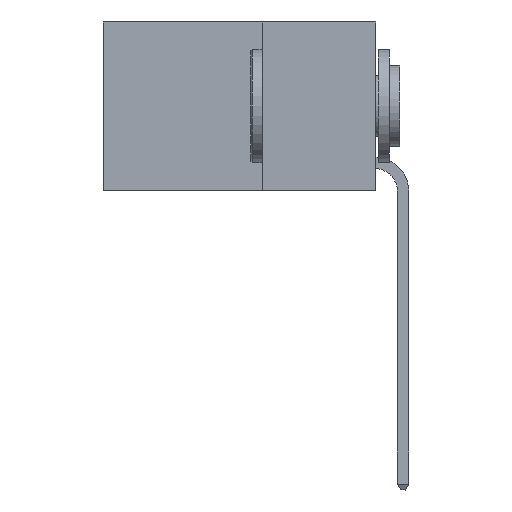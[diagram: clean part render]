
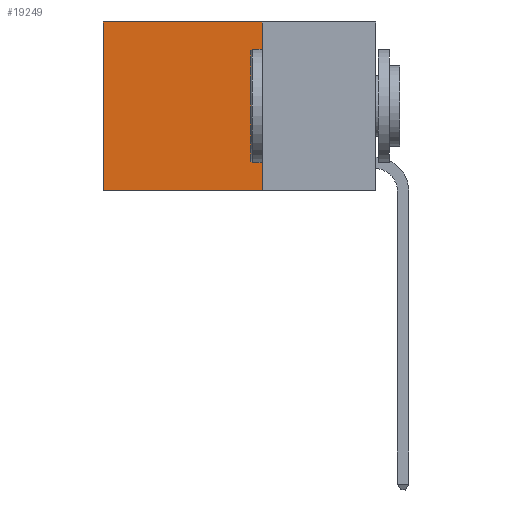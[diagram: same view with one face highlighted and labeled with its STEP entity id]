
A CAD part, left-side view. The second image highlights one B-rep face of the part: STEP entity #19249.
In plain terms, the highlighted planar face has unit normal (-1, 0, 0).
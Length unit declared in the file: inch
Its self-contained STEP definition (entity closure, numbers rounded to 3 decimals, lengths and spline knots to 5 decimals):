
#823 = VECTOR ( 'NONE', #17394, 39.37008 ) ;
#1607 = CARTESIAN_POINT ( 'NONE',  ( 0.2625, 0.25, -0.37 ) ) ;
#2812 = CARTESIAN_POINT ( 'NONE',  ( 0.2625, 0.6, 0. ) ) ;
#3030 = EDGE_CURVE ( 'NONE', #15011, #12267, #16130, .T. ) ;
#3965 = DIRECTION ( 'NONE',  ( 1., 0., 0. ) ) ;
#4365 = ORIENTED_EDGE ( 'NONE', *, *, #15243, .T. ) ;
#4957 = DIRECTION ( 'NONE',  ( 0., 1., 0. ) ) ;
#5393 = EDGE_CURVE ( 'NONE', #20760, #12267, #10944, .T. ) ;
#5872 = CARTESIAN_POINT ( 'NONE',  ( 0.2625, 0.25, 0. ) ) ;
#7926 = EDGE_CURVE ( 'NONE', #13585, #20760, #18431, .T. ) ;
#8277 = ORIENTED_EDGE ( 'NONE', *, *, #5393, .F. ) ;
#8427 = CARTESIAN_POINT ( 'NONE',  ( 0.2625, 0.25, 0. ) ) ;
#9033 = CARTESIAN_POINT ( 'NONE',  ( 0.2625, 0.6, 0. ) ) ;
#9902 = VECTOR ( 'NONE', #4957, 39.37008 ) ;
#10576 = VECTOR ( 'NONE', #16600, 39.37008 ) ;
#10944 = LINE ( 'NONE', #14856, #9902 ) ;
#12066 = ORIENTED_EDGE ( 'NONE', *, *, #3030, .T. ) ;
#12138 = ORIENTED_EDGE ( 'NONE', *, *, #7926, .F. ) ;
#12267 = VERTEX_POINT ( 'NONE', #15924 ) ;
#13585 = VERTEX_POINT ( 'NONE', #15942 ) ;
#13885 = CARTESIAN_POINT ( 'NONE',  ( 0.2625, 0.25, 0. ) ) ;
#14373 = FACE_OUTER_BOUND ( 'NONE', #16732, .T. ) ;
#14856 = CARTESIAN_POINT ( 'NONE',  ( 0.2625, 0.25, -0.37 ) ) ;
#15011 = VERTEX_POINT ( 'NONE', #2812 ) ;
#15243 = EDGE_CURVE ( 'NONE', #13585, #15011, #18701, .T. ) ;
#15514 = DIRECTION ( 'NONE',  ( 0., 0., -1. ) ) ;
#15924 = CARTESIAN_POINT ( 'NONE',  ( 0.2625, 0.6, -0.37 ) ) ;
#15942 = CARTESIAN_POINT ( 'NONE',  ( 0.2625, 0.25, 0. ) ) ;
#16130 = LINE ( 'NONE', #9033, #21243 ) ;
#16600 = DIRECTION ( 'NONE',  ( 0., 1., 0. ) ) ;
#16732 = EDGE_LOOP ( 'NONE', ( #12066, #8277, #12138, #4365 ) ) ;
#17394 = DIRECTION ( 'NONE',  ( 0., 0., -1. ) ) ;
#18431 = LINE ( 'NONE', #5872, #823 ) ;
#18699 = PLANE ( 'NONE',  #19033 ) ;
#18701 = LINE ( 'NONE', #8427, #10576 ) ;
#18818 = DIRECTION ( 'NONE',  ( 0., 0., -1. ) ) ;
#19033 = AXIS2_PLACEMENT_3D ( 'NONE', #13885, #3965, #15514 ) ;
#19249 = ADVANCED_FACE ( 'NONE', ( #14373 ), #18699, .F. ) ;
#20760 = VERTEX_POINT ( 'NONE', #1607 ) ;
#21243 = VECTOR ( 'NONE', #18818, 39.37008 ) ;
